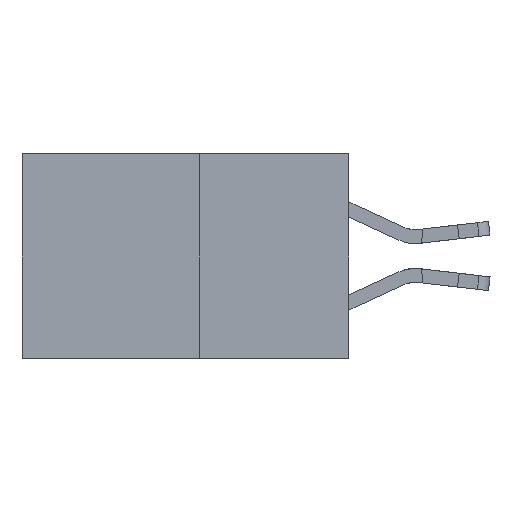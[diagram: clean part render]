
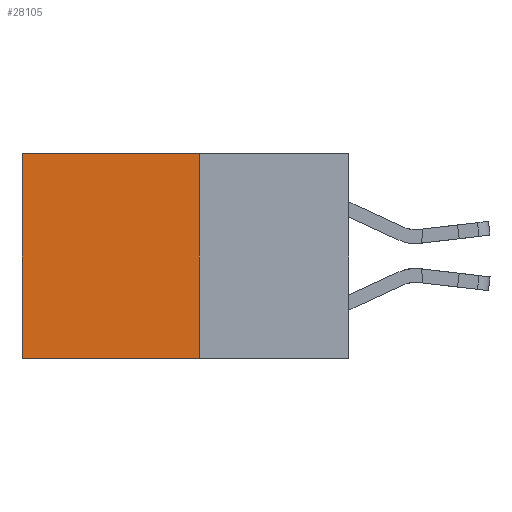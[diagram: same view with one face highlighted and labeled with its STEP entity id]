
A CAD part, left-side view. The second image highlights one B-rep face of the part: STEP entity #28105.
In plain terms, the highlighted planar face has unit normal (-1, 0, 0).
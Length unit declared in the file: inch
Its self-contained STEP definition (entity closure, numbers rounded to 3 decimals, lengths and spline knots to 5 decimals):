
#3030 = VERTEX_POINT ( 'NONE', #28307 ) ;
#3884 = VECTOR ( 'NONE', #17893, 39.37008 ) ;
#4311 = VECTOR ( 'NONE', #25310, 39.37008 ) ;
#4611 = CARTESIAN_POINT ( 'NONE',  ( 0.277, 0.27, 0. ) ) ;
#4852 = DIRECTION ( 'NONE',  ( 1., 0., 0. ) ) ;
#5123 = CARTESIAN_POINT ( 'NONE',  ( 0.277, 0.27, -0.37 ) ) ;
#8811 = CARTESIAN_POINT ( 'NONE',  ( 0.277, 0.59, -0.37 ) ) ;
#8823 = ORIENTED_EDGE ( 'NONE', *, *, #29886, .F. ) ;
#9791 = DIRECTION ( 'NONE',  ( 0., 0., -1. ) ) ;
#11619 = DIRECTION ( 'NONE',  ( 0., 1., 0. ) ) ;
#12743 = EDGE_CURVE ( 'NONE', #3030, #21171, #20896, .T. ) ;
#13116 = CARTESIAN_POINT ( 'NONE',  ( 0.277, 0.27, 0. ) ) ;
#13960 = VERTEX_POINT ( 'NONE', #13116 ) ;
#16157 = EDGE_CURVE ( 'NONE', #13960, #3030, #27402, .T. ) ;
#17585 = VECTOR ( 'NONE', #11619, 39.37008 ) ;
#17609 = ORIENTED_EDGE ( 'NONE', *, *, #18782, .F. ) ;
#17893 = DIRECTION ( 'NONE',  ( 0., 0., -1. ) ) ;
#18481 = CARTESIAN_POINT ( 'NONE',  ( 0.277, 0.27, -0.37 ) ) ;
#18703 = CARTESIAN_POINT ( 'NONE',  ( 0.277, 0.27, -0.37 ) ) ;
#18756 = CARTESIAN_POINT ( 'NONE',  ( 0.277, 0.27, -0.37 ) ) ;
#18782 = EDGE_CURVE ( 'NONE', #26836, #21171, #25154, .T. ) ;
#20896 = LINE ( 'NONE', #8811, #3884 ) ;
#21039 = DIRECTION ( 'NONE',  ( 0., 0., -1. ) ) ;
#21171 = VERTEX_POINT ( 'NONE', #21445 ) ;
#21445 = CARTESIAN_POINT ( 'NONE',  ( 0.277, 0.59, -0.37 ) ) ;
#21603 = LINE ( 'NONE', #5123, #26970 ) ;
#25154 = LINE ( 'NONE', #18481, #17585 ) ;
#25310 = DIRECTION ( 'NONE',  ( 0., 1., 0. ) ) ;
#26524 = EDGE_LOOP ( 'NONE', ( #27232, #17609, #8823, #29326 ) ) ;
#26836 = VERTEX_POINT ( 'NONE', #18756 ) ;
#26970 = VECTOR ( 'NONE', #9791, 39.37008 ) ;
#27083 = FACE_OUTER_BOUND ( 'NONE', #26524, .T. ) ;
#27232 = ORIENTED_EDGE ( 'NONE', *, *, #12743, .T. ) ;
#27402 = LINE ( 'NONE', #4611, #4311 ) ;
#27839 = PLANE ( 'NONE',  #28158 ) ;
#28105 = ADVANCED_FACE ( 'NONE', ( #27083 ), #27839, .F. ) ;
#28158 = AXIS2_PLACEMENT_3D ( 'NONE', #18703, #4852, #21039 ) ;
#28307 = CARTESIAN_POINT ( 'NONE',  ( 0.277, 0.59, 0. ) ) ;
#29326 = ORIENTED_EDGE ( 'NONE', *, *, #16157, .T. ) ;
#29886 = EDGE_CURVE ( 'NONE', #13960, #26836, #21603, .T. ) ;
